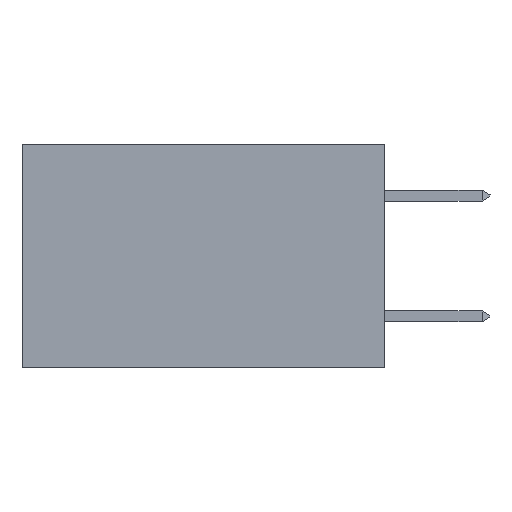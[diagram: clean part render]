
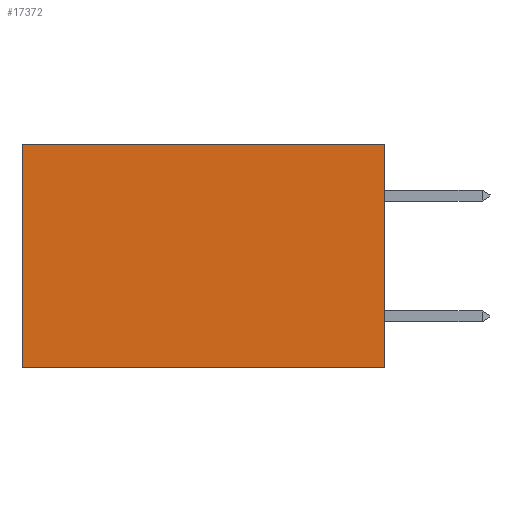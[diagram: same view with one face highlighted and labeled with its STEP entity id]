
A CAD part, left-side view. The second image highlights one B-rep face of the part: STEP entity #17372.
In plain terms, the highlighted planar face has unit normal (-1, 0, 0).
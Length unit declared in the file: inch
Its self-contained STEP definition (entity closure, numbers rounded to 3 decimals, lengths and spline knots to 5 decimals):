
#309 = CARTESIAN_POINT ( 'NONE',  ( 0.2875, 0.6, -0.37 ) ) ;
#447 = AXIS2_PLACEMENT_3D ( 'NONE', #17451, #6381, #3662 ) ;
#878 = CARTESIAN_POINT ( 'NONE',  ( 0.2875, 0., -0.37 ) ) ;
#2762 = CARTESIAN_POINT ( 'NONE',  ( 0.2875, 0., 0. ) ) ;
#3662 = DIRECTION ( 'NONE',  ( 0., 0., -1. ) ) ;
#4480 = CARTESIAN_POINT ( 'NONE',  ( 0.2875, 0., -0.37 ) ) ;
#5270 = VERTEX_POINT ( 'NONE', #16678 ) ;
#5417 = FACE_OUTER_BOUND ( 'NONE', #13945, .T. ) ;
#6381 = DIRECTION ( 'NONE',  ( 1., 0., 0. ) ) ;
#6439 = CARTESIAN_POINT ( 'NONE',  ( 0.2875, 0., 0. ) ) ;
#6766 = ORIENTED_EDGE ( 'NONE', *, *, #15979, .T. ) ;
#6790 = ORIENTED_EDGE ( 'NONE', *, *, #6960, .F. ) ;
#6960 = EDGE_CURVE ( 'NONE', #17596, #9896, #15154, .T. ) ;
#7196 = DIRECTION ( 'NONE',  ( 0., 1., 0. ) ) ;
#7431 = ORIENTED_EDGE ( 'NONE', *, *, #16389, .F. ) ;
#7819 = VECTOR ( 'NONE', #7196, 39.37008 ) ;
#8611 = CARTESIAN_POINT ( 'NONE',  ( 0.2875, 0.6, 0. ) ) ;
#9102 = VECTOR ( 'NONE', #16135, 39.37008 ) ;
#9246 = EDGE_CURVE ( 'NONE', #5270, #9892, #15142, .T. ) ;
#9892 = VERTEX_POINT ( 'NONE', #8611 ) ;
#9896 = VERTEX_POINT ( 'NONE', #309 ) ;
#11087 = ORIENTED_EDGE ( 'NONE', *, *, #9246, .T. ) ;
#11921 = LINE ( 'NONE', #12653, #9102 ) ;
#12653 = CARTESIAN_POINT ( 'NONE',  ( 0.2875, 0.6, 0. ) ) ;
#12802 = VECTOR ( 'NONE', #13395, 39.37008 ) ;
#13259 = PLANE ( 'NONE',  #447 ) ;
#13395 = DIRECTION ( 'NONE',  ( 0., 1., 0. ) ) ;
#13636 = DIRECTION ( 'NONE',  ( 0., 0., -1. ) ) ;
#13669 = LINE ( 'NONE', #6439, #15755 ) ;
#13945 = EDGE_LOOP ( 'NONE', ( #6766, #6790, #7431, #11087 ) ) ;
#15142 = LINE ( 'NONE', #2762, #7819 ) ;
#15154 = LINE ( 'NONE', #4480, #12802 ) ;
#15755 = VECTOR ( 'NONE', #13636, 39.37008 ) ;
#15979 = EDGE_CURVE ( 'NONE', #9892, #9896, #11921, .T. ) ;
#16135 = DIRECTION ( 'NONE',  ( 0., 0., -1. ) ) ;
#16389 = EDGE_CURVE ( 'NONE', #5270, #17596, #13669, .T. ) ;
#16678 = CARTESIAN_POINT ( 'NONE',  ( 0.2875, 0., 0. ) ) ;
#17372 = ADVANCED_FACE ( 'NONE', ( #5417 ), #13259, .F. ) ;
#17451 = CARTESIAN_POINT ( 'NONE',  ( 0.2875, 0., 0. ) ) ;
#17596 = VERTEX_POINT ( 'NONE', #878 ) ;
